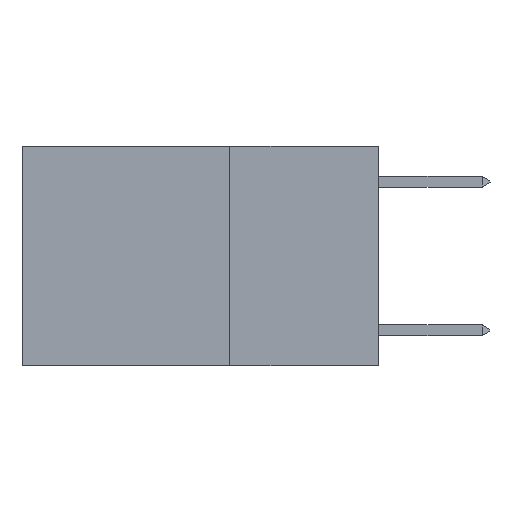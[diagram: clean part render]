
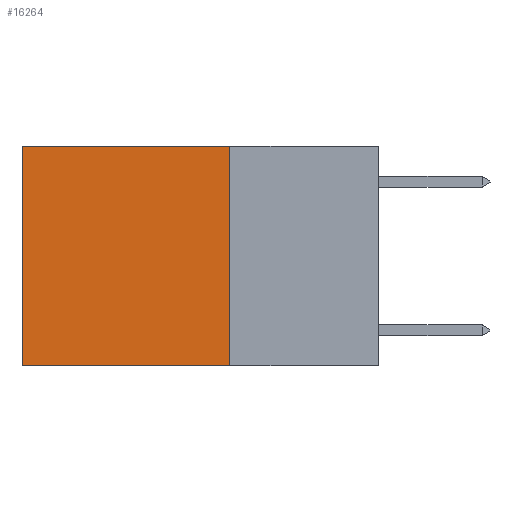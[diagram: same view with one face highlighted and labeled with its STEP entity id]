
A CAD part, left-side view. The second image highlights one B-rep face of the part: STEP entity #16264.
In plain terms, the highlighted planar face has unit normal (-1, 0, 0).
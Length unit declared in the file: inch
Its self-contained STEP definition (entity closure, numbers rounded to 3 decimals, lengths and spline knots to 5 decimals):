
#101 = VERTEX_POINT ( 'NONE', #23601 ) ;
#509 = EDGE_CURVE ( 'NONE', #101, #12225, #7880, .T. ) ;
#985 = EDGE_CURVE ( 'NONE', #3271, #101, #16304, .T. ) ;
#1719 = CARTESIAN_POINT ( 'NONE',  ( 0.2625, 0.25, 0. ) ) ;
#1839 = ORIENTED_EDGE ( 'NONE', *, *, #509, .F. ) ;
#2214 = EDGE_LOOP ( 'NONE', ( #2827, #1839, #15022, #13989 ) ) ;
#2827 = ORIENTED_EDGE ( 'NONE', *, *, #23938, .T. ) ;
#3271 = VERTEX_POINT ( 'NONE', #20298 ) ;
#4331 = VECTOR ( 'NONE', #18386, 39.37008 ) ;
#6040 = LINE ( 'NONE', #1719, #4331 ) ;
#6171 = CARTESIAN_POINT ( 'NONE',  ( 0.2625, 0.25, 0. ) ) ;
#6835 = CARTESIAN_POINT ( 'NONE',  ( 0.2625, 0.6, 0. ) ) ;
#7090 = CARTESIAN_POINT ( 'NONE',  ( 0.2625, 0.25, -0.37 ) ) ;
#7880 = LINE ( 'NONE', #7090, #14034 ) ;
#8387 = PLANE ( 'NONE',  #20682 ) ;
#8925 = EDGE_CURVE ( 'NONE', #3271, #9830, #6040, .T. ) ;
#9830 = VERTEX_POINT ( 'NONE', #15504 ) ;
#11015 = DIRECTION ( 'NONE',  ( 0., 0., -1. ) ) ;
#12225 = VERTEX_POINT ( 'NONE', #27132 ) ;
#13989 = ORIENTED_EDGE ( 'NONE', *, *, #8925, .T. ) ;
#14034 = VECTOR ( 'NONE', #17772, 39.37008 ) ;
#14609 = DIRECTION ( 'NONE',  ( 0., 0., -1. ) ) ;
#15022 = ORIENTED_EDGE ( 'NONE', *, *, #985, .F. ) ;
#15434 = VECTOR ( 'NONE', #26743, 39.37008 ) ;
#15504 = CARTESIAN_POINT ( 'NONE',  ( 0.2625, 0.6, 0. ) ) ;
#16079 = VECTOR ( 'NONE', #11015, 39.37008 ) ;
#16264 = ADVANCED_FACE ( 'NONE', ( #25486 ), #8387, .F. ) ;
#16304 = LINE ( 'NONE', #26341, #15434 ) ;
#16964 = LINE ( 'NONE', #6835, #16079 ) ;
#17772 = DIRECTION ( 'NONE',  ( 0., 1., 0. ) ) ;
#18386 = DIRECTION ( 'NONE',  ( 0., 1., 0. ) ) ;
#20298 = CARTESIAN_POINT ( 'NONE',  ( 0.2625, 0.25, 0. ) ) ;
#20615 = DIRECTION ( 'NONE',  ( 1., 0., 0. ) ) ;
#20682 = AXIS2_PLACEMENT_3D ( 'NONE', #6171, #20615, #14609 ) ;
#23601 = CARTESIAN_POINT ( 'NONE',  ( 0.2625, 0.25, -0.37 ) ) ;
#23938 = EDGE_CURVE ( 'NONE', #9830, #12225, #16964, .T. ) ;
#25486 = FACE_OUTER_BOUND ( 'NONE', #2214, .T. ) ;
#26341 = CARTESIAN_POINT ( 'NONE',  ( 0.2625, 0.25, 0. ) ) ;
#26743 = DIRECTION ( 'NONE',  ( 0., 0., -1. ) ) ;
#27132 = CARTESIAN_POINT ( 'NONE',  ( 0.2625, 0.6, -0.37 ) ) ;
